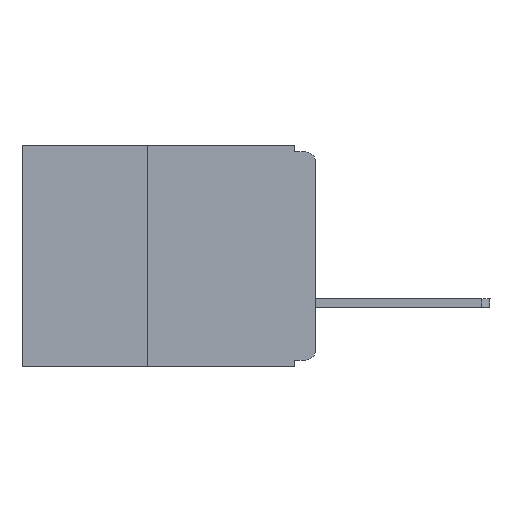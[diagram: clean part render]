
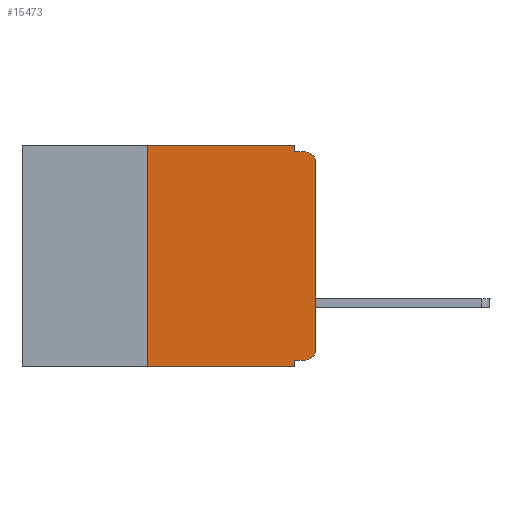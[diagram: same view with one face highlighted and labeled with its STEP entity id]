
A CAD part, left-side view. The second image highlights one B-rep face of the part: STEP entity #15473.
In plain terms, the highlighted planar face has unit normal (-1, 0, 0).
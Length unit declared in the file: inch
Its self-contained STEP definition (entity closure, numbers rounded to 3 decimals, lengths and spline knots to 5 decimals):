
#282 = LINE ( 'NONE', #15711, #5151 ) ;
#325 = EDGE_CURVE ( 'NONE', #6087, #10931, #6116, .T. ) ;
#353 = EDGE_CURVE ( 'NONE', #8625, #15626, #15125, .T. ) ;
#378 = ORIENTED_EDGE ( 'NONE', *, *, #13061, .F. ) ;
#657 = CARTESIAN_POINT ( 'NONE',  ( 0., 0.031, -0.33 ) ) ;
#711 = CARTESIAN_POINT ( 'NONE',  ( 0., 0.015, -0.32 ) ) ;
#1233 = CARTESIAN_POINT ( 'NONE',  ( 0., 0.031, 0. ) ) ;
#1501 = CARTESIAN_POINT ( 'NONE',  ( 0., 0.031, 0. ) ) ;
#1718 = DIRECTION ( 'NONE',  ( 0., 0., -1. ) ) ;
#2099 = DIRECTION ( 'NONE',  ( 0., -1., 0. ) ) ;
#2216 = VERTEX_POINT ( 'NONE', #5233 ) ;
#2819 = VECTOR ( 'NONE', #2099, 39.37008 ) ;
#3105 = CARTESIAN_POINT ( 'NONE',  ( 0., 0.015, -0.01 ) ) ;
#3193 = ORIENTED_EDGE ( 'NONE', *, *, #13669, .T. ) ;
#3339 = ORIENTED_EDGE ( 'NONE', *, *, #4721, .T. ) ;
#3493 = ORIENTED_EDGE ( 'NONE', *, *, #13915, .F. ) ;
#3568 = DIRECTION ( 'NONE',  ( 0., 0., 1. ) ) ;
#3615 = EDGE_CURVE ( 'NONE', #15626, #2216, #16029, .T. ) ;
#3658 = VECTOR ( 'NONE', #6187, 39.37008 ) ;
#3742 = DIRECTION ( 'NONE',  ( 0., 0., -1. ) ) ;
#3764 = CARTESIAN_POINT ( 'NONE',  ( 0., 0.031, -0.33 ) ) ;
#3885 = ORIENTED_EDGE ( 'NONE', *, *, #4931, .F. ) ;
#4008 = DIRECTION ( 'NONE',  ( 0., -1., 0. ) ) ;
#4094 = VECTOR ( 'NONE', #3568, 39.37008 ) ;
#4394 = DIRECTION ( 'NONE',  ( 0., 1., 0. ) ) ;
#4461 = CARTESIAN_POINT ( 'NONE',  ( 0., 0.015, -0.025 ) ) ;
#4634 = LINE ( 'NONE', #1233, #3658 ) ;
#4721 = EDGE_CURVE ( 'NONE', #2216, #10931, #9912, .T. ) ;
#4931 = EDGE_CURVE ( 'NONE', #5029, #6087, #4634, .T. ) ;
#4997 = CARTESIAN_POINT ( 'NONE',  ( 0., 0.015, -0.305 ) ) ;
#5029 = VERTEX_POINT ( 'NONE', #1501 ) ;
#5095 = AXIS2_PLACEMENT_3D ( 'NONE', #4461, #6860, #9483 ) ;
#5151 = VECTOR ( 'NONE', #4394, 39.37008 ) ;
#5233 = CARTESIAN_POINT ( 'NONE',  ( 0., 0., -0.025 ) ) ;
#5310 = VERTEX_POINT ( 'NONE', #6998 ) ;
#5747 = CARTESIAN_POINT ( 'NONE',  ( 0., 0.25, -0.33 ) ) ;
#6087 = VERTEX_POINT ( 'NONE', #7749 ) ;
#6116 = LINE ( 'NONE', #13536, #2819 ) ;
#6187 = DIRECTION ( 'NONE',  ( 0., 0., -1. ) ) ;
#6834 = ORIENTED_EDGE ( 'NONE', *, *, #11501, .F. ) ;
#6860 = DIRECTION ( 'NONE',  ( -1., 0., 0. ) ) ;
#6998 = CARTESIAN_POINT ( 'NONE',  ( 0., 0.031, -0.32 ) ) ;
#7749 = CARTESIAN_POINT ( 'NONE',  ( 0., 0.031, -0.01 ) ) ;
#7804 = AXIS2_PLACEMENT_3D ( 'NONE', #4997, #13583, #3742 ) ;
#7810 = LINE ( 'NONE', #12930, #11758 ) ;
#8290 = CARTESIAN_POINT ( 'NONE',  ( 0., 0., -0.305 ) ) ;
#8494 = DIRECTION ( 'NONE',  ( 0., 0., 1. ) ) ;
#8625 = VERTEX_POINT ( 'NONE', #711 ) ;
#8646 = CARTESIAN_POINT ( 'NONE',  ( 0., 0.25, -0.33 ) ) ;
#8850 = AXIS2_PLACEMENT_3D ( 'NONE', #9201, #14246, #1718 ) ;
#9189 = VERTEX_POINT ( 'NONE', #8646 ) ;
#9201 = CARTESIAN_POINT ( 'NONE',  ( 0., 0.437, 0. ) ) ;
#9274 = VERTEX_POINT ( 'NONE', #3764 ) ;
#9483 = DIRECTION ( 'NONE',  ( 0., 0., -1. ) ) ;
#9690 = ORIENTED_EDGE ( 'NONE', *, *, #353, .T. ) ;
#9735 = FACE_OUTER_BOUND ( 'NONE', #14994, .T. ) ;
#9912 = CIRCLE ( 'NONE', #5095, 0.015 ) ;
#10692 = VERTEX_POINT ( 'NONE', #15347 ) ;
#10767 = LINE ( 'NONE', #657, #15295 ) ;
#10931 = VERTEX_POINT ( 'NONE', #3105 ) ;
#10940 = CARTESIAN_POINT ( 'NONE',  ( 0., 0., 0. ) ) ;
#11501 = EDGE_CURVE ( 'NONE', #8625, #5310, #282, .T. ) ;
#11758 = VECTOR ( 'NONE', #4008, 39.37008 ) ;
#11796 = EDGE_CURVE ( 'NONE', #9189, #10692, #15895, .T. ) ;
#12327 = VECTOR ( 'NONE', #15849, 39.37008 ) ;
#12878 = ORIENTED_EDGE ( 'NONE', *, *, #325, .F. ) ;
#12930 = CARTESIAN_POINT ( 'NONE',  ( 0., 0.437, 0. ) ) ;
#13061 = EDGE_CURVE ( 'NONE', #10692, #5029, #7810, .T. ) ;
#13217 = DIRECTION ( 'NONE',  ( 0., 0., -1. ) ) ;
#13444 = CARTESIAN_POINT ( 'NONE',  ( 0., 0.437, -0.33 ) ) ;
#13536 = CARTESIAN_POINT ( 'NONE',  ( 0., 0., -0.01 ) ) ;
#13583 = DIRECTION ( 'NONE',  ( -1., 0., 0. ) ) ;
#13669 = EDGE_CURVE ( 'NONE', #9189, #9274, #14478, .T. ) ;
#13915 = EDGE_CURVE ( 'NONE', #5310, #9274, #10767, .T. ) ;
#14191 = PLANE ( 'NONE',  #8850 ) ;
#14246 = DIRECTION ( 'NONE',  ( 1., 0., 0. ) ) ;
#14478 = LINE ( 'NONE', #13444, #12327 ) ;
#14531 = VECTOR ( 'NONE', #8494, 39.37008 ) ;
#14915 = ORIENTED_EDGE ( 'NONE', *, *, #3615, .T. ) ;
#14994 = EDGE_LOOP ( 'NONE', ( #14915, #3339, #12878, #3885, #378, #15635, #3193, #3493, #6834, #9690 ) ) ;
#15125 = CIRCLE ( 'NONE', #7804, 0.015 ) ;
#15295 = VECTOR ( 'NONE', #13217, 39.37008 ) ;
#15347 = CARTESIAN_POINT ( 'NONE',  ( 0., 0.25, 0. ) ) ;
#15473 = ADVANCED_FACE ( 'NONE', ( #9735 ), #14191, .F. ) ;
#15626 = VERTEX_POINT ( 'NONE', #8290 ) ;
#15635 = ORIENTED_EDGE ( 'NONE', *, *, #11796, .F. ) ;
#15711 = CARTESIAN_POINT ( 'NONE',  ( 0., 0., -0.32 ) ) ;
#15849 = DIRECTION ( 'NONE',  ( 0., -1., 0. ) ) ;
#15895 = LINE ( 'NONE', #5747, #14531 ) ;
#16029 = LINE ( 'NONE', #10940, #4094 ) ;
